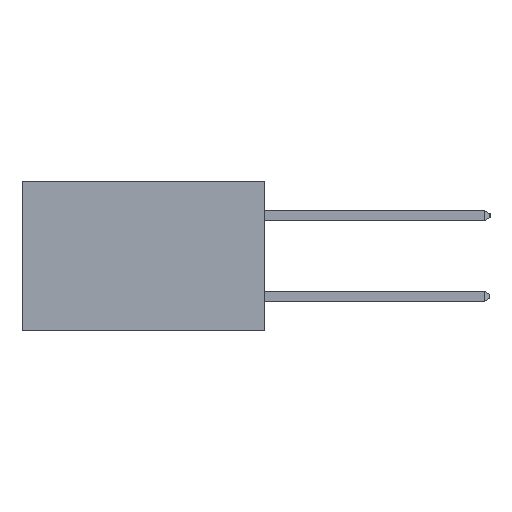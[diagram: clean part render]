
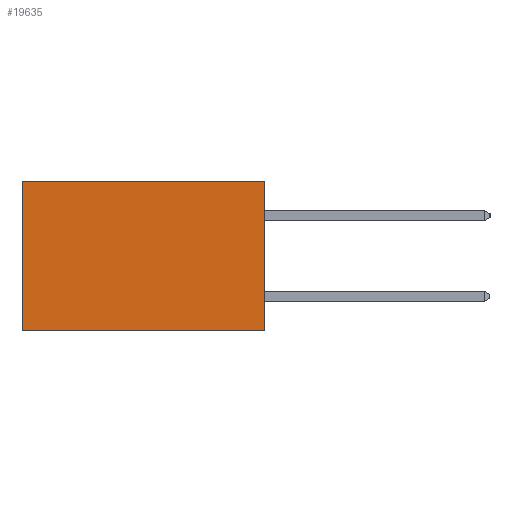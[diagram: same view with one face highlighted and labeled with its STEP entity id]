
A CAD part, left-side view. The second image highlights one B-rep face of the part: STEP entity #19635.
In plain terms, the highlighted planar face has unit normal (-1, 0, 0).
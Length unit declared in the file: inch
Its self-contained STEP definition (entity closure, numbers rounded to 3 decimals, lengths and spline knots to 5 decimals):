
#374 = AXIS2_PLACEMENT_3D ( 'NONE', #18961, #20991, #8862 ) ;
#1171 = ORIENTED_EDGE ( 'NONE', *, *, #20545, .T. ) ;
#2340 = VECTOR ( 'NONE', #17599, 39.37008 ) ;
#2863 = ORIENTED_EDGE ( 'NONE', *, *, #21170, .F. ) ;
#5467 = CARTESIAN_POINT ( 'NONE',  ( 0.2615, 0., 0. ) ) ;
#5717 = ORIENTED_EDGE ( 'NONE', *, *, #22511, .T. ) ;
#5722 = DIRECTION ( 'NONE',  ( 0., 1., 0. ) ) ;
#8765 = CARTESIAN_POINT ( 'NONE',  ( 0.2615, 0.6, -0.37 ) ) ;
#8862 = DIRECTION ( 'NONE',  ( 0., 0., -1. ) ) ;
#8867 = VECTOR ( 'NONE', #23803, 39.37008 ) ;
#9634 = CARTESIAN_POINT ( 'NONE',  ( 0.2615, 0.6, -0.37 ) ) ;
#11327 = VERTEX_POINT ( 'NONE', #8765 ) ;
#12171 = VECTOR ( 'NONE', #5722, 39.37008 ) ;
#12511 = ORIENTED_EDGE ( 'NONE', *, *, #12922, .F. ) ;
#12634 = VERTEX_POINT ( 'NONE', #20748 ) ;
#12922 = EDGE_CURVE ( 'NONE', #12634, #11327, #17553, .T. ) ;
#13621 = LINE ( 'NONE', #9634, #8867 ) ;
#14024 = LINE ( 'NONE', #17387, #24818 ) ;
#14872 = PLANE ( 'NONE',  #374 ) ;
#14972 = EDGE_LOOP ( 'NONE', ( #5717, #12511, #2863, #1171 ) ) ;
#15386 = CARTESIAN_POINT ( 'NONE',  ( 0.2615, 0., 0. ) ) ;
#17051 = VERTEX_POINT ( 'NONE', #15386 ) ;
#17076 = VERTEX_POINT ( 'NONE', #23553 ) ;
#17387 = CARTESIAN_POINT ( 'NONE',  ( 0.2615, 0., -0.37 ) ) ;
#17553 = LINE ( 'NONE', #23853, #12171 ) ;
#17599 = DIRECTION ( 'NONE',  ( 0., 1., 0. ) ) ;
#18961 = CARTESIAN_POINT ( 'NONE',  ( 0.2615, 0., -0.37 ) ) ;
#19397 = DIRECTION ( 'NONE',  ( 0., 0., -1. ) ) ;
#19635 = ADVANCED_FACE ( 'NONE', ( #23289 ), #14872, .F. ) ;
#20545 = EDGE_CURVE ( 'NONE', #17051, #17076, #23237, .T. ) ;
#20748 = CARTESIAN_POINT ( 'NONE',  ( 0.2615, 0., -0.37 ) ) ;
#20991 = DIRECTION ( 'NONE',  ( 1., 0., 0. ) ) ;
#21170 = EDGE_CURVE ( 'NONE', #17051, #12634, #14024, .T. ) ;
#22511 = EDGE_CURVE ( 'NONE', #17076, #11327, #13621, .T. ) ;
#23237 = LINE ( 'NONE', #5467, #2340 ) ;
#23289 = FACE_OUTER_BOUND ( 'NONE', #14972, .T. ) ;
#23553 = CARTESIAN_POINT ( 'NONE',  ( 0.2615, 0.6, 0. ) ) ;
#23803 = DIRECTION ( 'NONE',  ( 0., 0., -1. ) ) ;
#23853 = CARTESIAN_POINT ( 'NONE',  ( 0.2615, 0., -0.37 ) ) ;
#24818 = VECTOR ( 'NONE', #19397, 39.37008 ) ;
